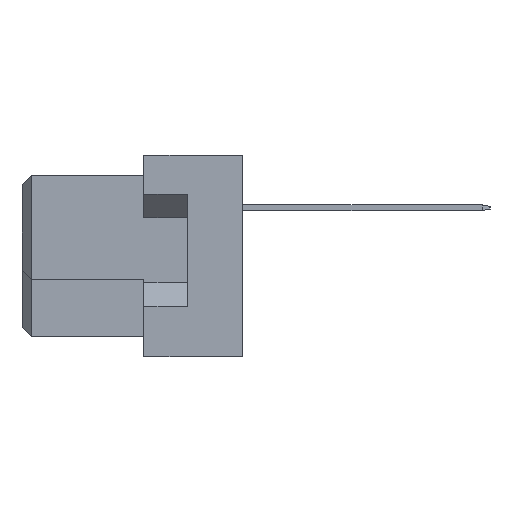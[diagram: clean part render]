
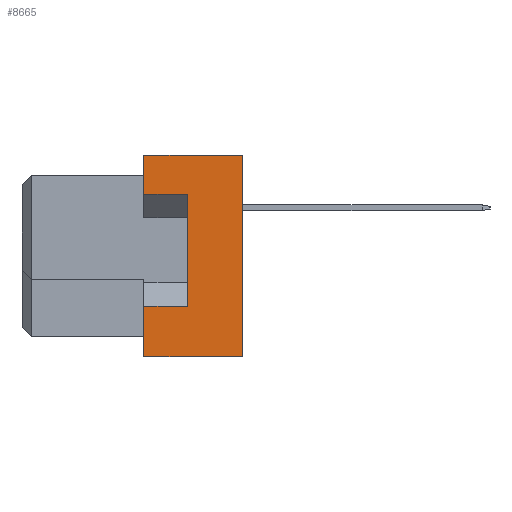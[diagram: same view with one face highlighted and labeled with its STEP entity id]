
A CAD part, left-side view. The second image highlights one B-rep face of the part: STEP entity #8665.
In plain terms, the highlighted planar face has unit normal (-1, 0, 0).
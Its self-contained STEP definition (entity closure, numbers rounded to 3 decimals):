
#1337 = CARTESIAN_POINT ( 'NONE',  ( -47.5, -11.6, -5.3 ) ) ;
#1801 = VECTOR ( 'NONE', #23219, 1000. ) ;
#1880 = CARTESIAN_POINT ( 'NONE',  ( -47.5, -8.7, -2.65 ) ) ;
#2227 = DIRECTION ( 'NONE',  ( 0., 1., 0. ) ) ;
#2279 = FACE_OUTER_BOUND ( 'NONE', #32863, .T. ) ;
#3570 = DIRECTION ( 'NONE',  ( 0., 0., 1. ) ) ;
#4441 = DIRECTION ( 'NONE',  ( 0., 0., 1. ) ) ;
#5224 = VECTOR ( 'NONE', #32680, 1000. ) ;
#6023 = VECTOR ( 'NONE', #4441, 1000. ) ;
#6584 = ORIENTED_EDGE ( 'NONE', *, *, #16977, .T. ) ;
#6831 = LINE ( 'NONE', #30022, #37152 ) ;
#7483 = EDGE_CURVE ( 'NONE', #12534, #28026, #18634, .T. ) ;
#7672 = CARTESIAN_POINT ( 'NONE',  ( -47.5, -6.4, -5.3 ) ) ;
#7794 = ORIENTED_EDGE ( 'NONE', *, *, #29940, .F. ) ;
#8526 = LINE ( 'NONE', #34985, #1801 ) ;
#8665 = ADVANCED_FACE ( 'NONE', ( #2279 ), #28931, .T. ) ;
#9193 = VERTEX_POINT ( 'NONE', #1337 ) ;
#10093 = CARTESIAN_POINT ( 'NONE',  ( -47.5, -6.4, 5.3 ) ) ;
#10748 = CARTESIAN_POINT ( 'NONE',  ( -47.5, -8.7, 3.25 ) ) ;
#11522 = LINE ( 'NONE', #7672, #22558 ) ;
#12534 = VERTEX_POINT ( 'NONE', #1880 ) ;
#12610 = EDGE_CURVE ( 'NONE', #24022, #28026, #11522, .T. ) ;
#12622 = CARTESIAN_POINT ( 'NONE',  ( -47.5, -8.7, -2.65 ) ) ;
#14842 = CARTESIAN_POINT ( 'NONE',  ( -47.5, -6.4, 3.25 ) ) ;
#15423 = EDGE_CURVE ( 'NONE', #23646, #20987, #8526, .T. ) ;
#16732 = ORIENTED_EDGE ( 'NONE', *, *, #15423, .F. ) ;
#16977 = EDGE_CURVE ( 'NONE', #21121, #18789, #37218, .T. ) ;
#17355 = DIRECTION ( 'NONE',  ( 0., 0., 1. ) ) ;
#18634 = LINE ( 'NONE', #12622, #28985 ) ;
#18789 = VERTEX_POINT ( 'NONE', #10093 ) ;
#19934 = ORIENTED_EDGE ( 'NONE', *, *, #21871, .F. ) ;
#20172 = ORIENTED_EDGE ( 'NONE', *, *, #34730, .F. ) ;
#20987 = VERTEX_POINT ( 'NONE', #14842 ) ;
#21121 = VERTEX_POINT ( 'NONE', #28709 ) ;
#21566 = CARTESIAN_POINT ( 'NONE',  ( -47.5, -6.4, -2.65 ) ) ;
#21871 = EDGE_CURVE ( 'NONE', #12534, #23646, #27429, .T. ) ;
#22155 = ORIENTED_EDGE ( 'NONE', *, *, #12610, .F. ) ;
#22558 = VECTOR ( 'NONE', #22755, 1000. ) ;
#22755 = DIRECTION ( 'NONE',  ( 0., 0., 1. ) ) ;
#23219 = DIRECTION ( 'NONE',  ( 0., 1., 0. ) ) ;
#23408 = ORIENTED_EDGE ( 'NONE', *, *, #7483, .T. ) ;
#23646 = VERTEX_POINT ( 'NONE', #10748 ) ;
#24022 = VERTEX_POINT ( 'NONE', #28109 ) ;
#25266 = DIRECTION ( 'NONE',  ( 0., 1., 0. ) ) ;
#25310 = VECTOR ( 'NONE', #25266, 1000. ) ;
#27045 = EDGE_CURVE ( 'NONE', #9193, #21121, #6831, .T. ) ;
#27268 = LINE ( 'NONE', #30347, #5224 ) ;
#27429 = LINE ( 'NONE', #36323, #6023 ) ;
#28026 = VERTEX_POINT ( 'NONE', #21566 ) ;
#28109 = CARTESIAN_POINT ( 'NONE',  ( -47.5, -6.4, -5.3 ) ) ;
#28162 = CARTESIAN_POINT ( 'NONE',  ( -47.5, -11.6, 5.3 ) ) ;
#28709 = CARTESIAN_POINT ( 'NONE',  ( -47.5, -11.6, 5.3 ) ) ;
#28931 = PLANE ( 'NONE',  #32637 ) ;
#28985 = VECTOR ( 'NONE', #30218, 1000. ) ;
#29940 = EDGE_CURVE ( 'NONE', #20987, #18789, #27268, .T. ) ;
#30022 = CARTESIAN_POINT ( 'NONE',  ( -47.5, -11.6, 5.3 ) ) ;
#30218 = DIRECTION ( 'NONE',  ( 0., 1., 0. ) ) ;
#30347 = CARTESIAN_POINT ( 'NONE',  ( -47.5, -6.4, -5.3 ) ) ;
#31832 = CARTESIAN_POINT ( 'NONE',  ( -47.5, -11.6, 5.3 ) ) ;
#32637 = AXIS2_PLACEMENT_3D ( 'NONE', #31832, #34338, #17355 ) ;
#32680 = DIRECTION ( 'NONE',  ( 0., 0., 1. ) ) ;
#32863 = EDGE_LOOP ( 'NONE', ( #23408, #22155, #20172, #34924, #6584, #7794, #16732, #19934 ) ) ;
#34338 = DIRECTION ( 'NONE',  ( -1., 0., 0. ) ) ;
#34666 = CARTESIAN_POINT ( 'NONE',  ( -47.5, -11.6, -5.3 ) ) ;
#34730 = EDGE_CURVE ( 'NONE', #9193, #24022, #38145, .T. ) ;
#34924 = ORIENTED_EDGE ( 'NONE', *, *, #27045, .T. ) ;
#34985 = CARTESIAN_POINT ( 'NONE',  ( -47.5, -8.7, 3.25 ) ) ;
#36190 = VECTOR ( 'NONE', #2227, 1000. ) ;
#36323 = CARTESIAN_POINT ( 'NONE',  ( -47.5, -8.7, -2.65 ) ) ;
#37152 = VECTOR ( 'NONE', #3570, 1000. ) ;
#37218 = LINE ( 'NONE', #28162, #25310 ) ;
#38145 = LINE ( 'NONE', #34666, #36190 ) ;
